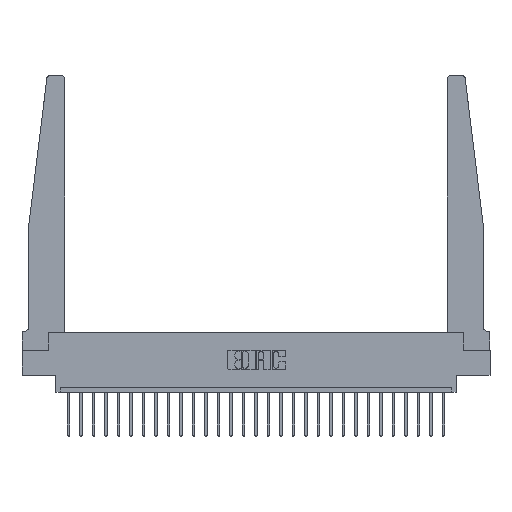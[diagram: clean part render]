
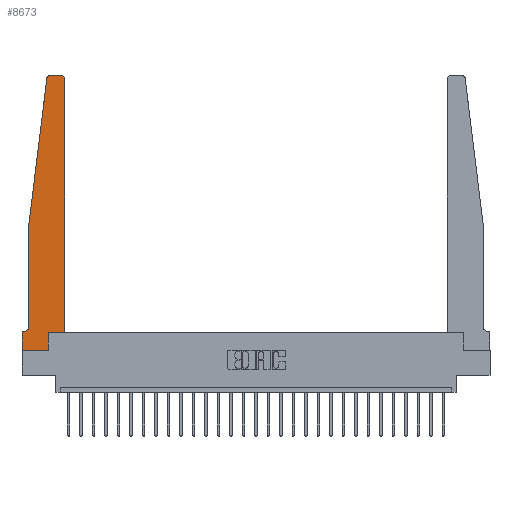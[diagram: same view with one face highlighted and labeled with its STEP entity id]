
A CAD part, top view. The second image highlights one B-rep face of the part: STEP entity #8673.
In plain terms, the highlighted planar face has unit normal (0, 0, 1).
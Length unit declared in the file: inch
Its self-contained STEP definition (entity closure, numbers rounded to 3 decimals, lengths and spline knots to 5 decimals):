
#124 = LINE ( 'NONE', #8013, #25087 ) ;
#150 = VECTOR ( 'NONE', #17885, 39.37008 ) ;
#154 = AXIS2_PLACEMENT_3D ( 'NONE', #1578, #15546, #21479 ) ;
#185 = CARTESIAN_POINT ( 'NONE',  ( 0.065, 0.2375, 0.37 ) ) ;
#754 = VECTOR ( 'NONE', #20191, 39.37008 ) ;
#1578 = CARTESIAN_POINT ( 'NONE',  ( 0., 0.1875, 0.37 ) ) ;
#1702 = PLANE ( 'NONE',  #154 ) ;
#1723 = DIRECTION ( 'NONE',  ( 0., 1., 0. ) ) ;
#1872 = LINE ( 'NONE', #12015, #10400 ) ;
#2004 = EDGE_LOOP ( 'NONE', ( #9803, #23439, #15834, #10011, #25104, #14544, #13526, #7013, #6945, #16395, #19140, #10216 ) ) ;
#2268 = CARTESIAN_POINT ( 'NONE',  ( 0.2605, 0.18, 0.37 ) ) ;
#3166 = VECTOR ( 'NONE', #4635, 39.37008 ) ;
#3466 = EDGE_CURVE ( 'NONE', #25161, #21791, #124, .T. ) ;
#3527 = VERTEX_POINT ( 'NONE', #5910 ) ;
#4030 = LINE ( 'NONE', #7855, #20441 ) ;
#4635 = DIRECTION ( 'NONE',  ( 1., 0., 0. ) ) ;
#5151 = EDGE_CURVE ( 'NONE', #15692, #25161, #24430, .T. ) ;
#5496 = CARTESIAN_POINT ( 'NONE',  ( 0., 0., 0.37 ) ) ;
#5618 = VERTEX_POINT ( 'NONE', #9628 ) ;
#5868 = DIRECTION ( 'NONE',  ( -1., 0., 0. ) ) ;
#5887 = LINE ( 'NONE', #24092, #150 ) ;
#5910 = CARTESIAN_POINT ( 'NONE',  ( 0.395, 2.75, 0.37 ) ) ;
#6393 = AXIS2_PLACEMENT_3D ( 'NONE', #17388, #13429, #23739 ) ;
#6864 = CARTESIAN_POINT ( 'NONE',  ( 0.2605, 0.18, 0.37 ) ) ;
#6945 = ORIENTED_EDGE ( 'NONE', *, *, #22177, .T. ) ;
#7013 = ORIENTED_EDGE ( 'NONE', *, *, #17796, .T. ) ;
#7057 = DIRECTION ( 'NONE',  ( -1., 0., 0. ) ) ;
#7163 = DIRECTION ( 'NONE',  ( 1., 0., 0. ) ) ;
#7855 = CARTESIAN_POINT ( 'NONE',  ( 0.25, 2.75, 0.37 ) ) ;
#7976 = DIRECTION ( 'NONE',  ( -1., 0., 0. ) ) ;
#8013 = CARTESIAN_POINT ( 'NONE',  ( 0.065, 1.25, 0.37 ) ) ;
#8290 = VECTOR ( 'NONE', #10945, 39.37008 ) ;
#8320 = CARTESIAN_POINT ( 'NONE',  ( 0., 0., 0.37 ) ) ;
#8554 = CARTESIAN_POINT ( 'NONE',  ( 0.27653, 2.75, 0.37 ) ) ;
#8673 = ADVANCED_FACE ( 'NONE', ( #11455 ), #1702, .T. ) ;
#9099 = LINE ( 'NONE', #20990, #3166 ) ;
#9362 = CARTESIAN_POINT ( 'NONE',  ( 0.425, 0.18, 0.37 ) ) ;
#9556 = EDGE_CURVE ( 'NONE', #5618, #19432, #23888, .T. ) ;
#9581 = VERTEX_POINT ( 'NONE', #9625 ) ;
#9586 = AXIS2_PLACEMENT_3D ( 'NONE', #12993, #14846, #7057 ) ;
#9625 = CARTESIAN_POINT ( 'NONE',  ( 0., 0.1875, 0.37 ) ) ;
#9628 = CARTESIAN_POINT ( 'NONE',  ( 0.425, 0.18, 0.37 ) ) ;
#9803 = ORIENTED_EDGE ( 'NONE', *, *, #18367, .T. ) ;
#9950 = CARTESIAN_POINT ( 'NONE',  ( 0.065, 0.1875, 0.37 ) ) ;
#10011 = ORIENTED_EDGE ( 'NONE', *, *, #20409, .T. ) ;
#10216 = ORIENTED_EDGE ( 'NONE', *, *, #13007, .T. ) ;
#10400 = VECTOR ( 'NONE', #15573, 39.37008 ) ;
#10430 = VERTEX_POINT ( 'NONE', #185 ) ;
#10945 = DIRECTION ( 'NONE',  ( 0., 1., 0. ) ) ;
#11455 = FACE_OUTER_BOUND ( 'NONE', #2004, .T. ) ;
#11793 = VERTEX_POINT ( 'NONE', #24856 ) ;
#11809 = LINE ( 'NONE', #9950, #12386 ) ;
#12015 = CARTESIAN_POINT ( 'NONE',  ( 0.065, 1.25, 0.37 ) ) ;
#12386 = VECTOR ( 'NONE', #5868, 39.37008 ) ;
#12993 = CARTESIAN_POINT ( 'NONE',  ( 0.015, 0.2375, 0.37 ) ) ;
#13007 = EDGE_CURVE ( 'NONE', #19432, #3527, #22009, .T. ) ;
#13429 = DIRECTION ( 'NONE',  ( 0., 0., 1. ) ) ;
#13526 = ORIENTED_EDGE ( 'NONE', *, *, #20871, .T. ) ;
#13634 = EDGE_CURVE ( 'NONE', #25798, #5618, #5887, .T. ) ;
#14544 = ORIENTED_EDGE ( 'NONE', *, *, #16645, .T. ) ;
#14650 = CIRCLE ( 'NONE', #9586, 0.05 ) ;
#14838 = CARTESIAN_POINT ( 'NONE',  ( 0.24675, 2.72367, 0.37 ) ) ;
#14846 = DIRECTION ( 'NONE',  ( 0., 0., -1. ) ) ;
#15546 = DIRECTION ( 'NONE',  ( 0., 0., 1. ) ) ;
#15573 = DIRECTION ( 'NONE',  ( 0., -1., 0. ) ) ;
#15692 = VERTEX_POINT ( 'NONE', #8554 ) ;
#15834 = ORIENTED_EDGE ( 'NONE', *, *, #3466, .T. ) ;
#16076 = VERTEX_POINT ( 'NONE', #5496 ) ;
#16162 = VECTOR ( 'NONE', #1723, 39.37008 ) ;
#16395 = ORIENTED_EDGE ( 'NONE', *, *, #13634, .T. ) ;
#16645 = EDGE_CURVE ( 'NONE', #11793, #9581, #11809, .T. ) ;
#16879 = LINE ( 'NONE', #6864, #8290 ) ;
#17055 = DIRECTION ( 'NONE',  ( 0., 0., 1. ) ) ;
#17122 = CARTESIAN_POINT ( 'NONE',  ( 0.425, 2.72, 0.37 ) ) ;
#17388 = CARTESIAN_POINT ( 'NONE',  ( 0.395, 2.72, 0.37 ) ) ;
#17796 = EDGE_CURVE ( 'NONE', #16076, #25856, #9099, .T. ) ;
#17885 = DIRECTION ( 'NONE',  ( 1., 0., 0. ) ) ;
#18367 = EDGE_CURVE ( 'NONE', #3527, #15692, #4030, .T. ) ;
#18595 = LINE ( 'NONE', #8320, #754 ) ;
#18950 = AXIS2_PLACEMENT_3D ( 'NONE', #19164, #17055, #7163 ) ;
#19140 = ORIENTED_EDGE ( 'NONE', *, *, #9556, .T. ) ;
#19164 = CARTESIAN_POINT ( 'NONE',  ( 0.27653, 2.72, 0.37 ) ) ;
#19432 = VERTEX_POINT ( 'NONE', #17122 ) ;
#20191 = DIRECTION ( 'NONE',  ( 0., -1., 0. ) ) ;
#20409 = EDGE_CURVE ( 'NONE', #21791, #10430, #1872, .T. ) ;
#20441 = VECTOR ( 'NONE', #7976, 39.37008 ) ;
#20871 = EDGE_CURVE ( 'NONE', #9581, #16076, #18595, .T. ) ;
#20990 = CARTESIAN_POINT ( 'NONE',  ( 0., 0., 0.37 ) ) ;
#21479 = DIRECTION ( 'NONE',  ( 1., 0., 0. ) ) ;
#21791 = VERTEX_POINT ( 'NONE', #25109 ) ;
#22009 = CIRCLE ( 'NONE', #6393, 0.03 ) ;
#22149 = DIRECTION ( 'NONE',  ( -0.122, -0.992, 0. ) ) ;
#22177 = EDGE_CURVE ( 'NONE', #25856, #25798, #16879, .T. ) ;
#22959 = CARTESIAN_POINT ( 'NONE',  ( 0.2605, 0., 0.37 ) ) ;
#23044 = EDGE_CURVE ( 'NONE', #10430, #11793, #14650, .T. ) ;
#23439 = ORIENTED_EDGE ( 'NONE', *, *, #5151, .T. ) ;
#23739 = DIRECTION ( 'NONE',  ( 1., 0., 0. ) ) ;
#23888 = LINE ( 'NONE', #9362, #16162 ) ;
#24092 = CARTESIAN_POINT ( 'NONE',  ( 0.425, 0.18, 0.37 ) ) ;
#24430 = CIRCLE ( 'NONE', #18950, 0.03 ) ;
#24856 = CARTESIAN_POINT ( 'NONE',  ( 0.015, 0.1875, 0.37 ) ) ;
#25087 = VECTOR ( 'NONE', #22149, 39.37008 ) ;
#25104 = ORIENTED_EDGE ( 'NONE', *, *, #23044, .T. ) ;
#25109 = CARTESIAN_POINT ( 'NONE',  ( 0.065, 1.25, 0.37 ) ) ;
#25161 = VERTEX_POINT ( 'NONE', #14838 ) ;
#25798 = VERTEX_POINT ( 'NONE', #2268 ) ;
#25856 = VERTEX_POINT ( 'NONE', #22959 ) ;
